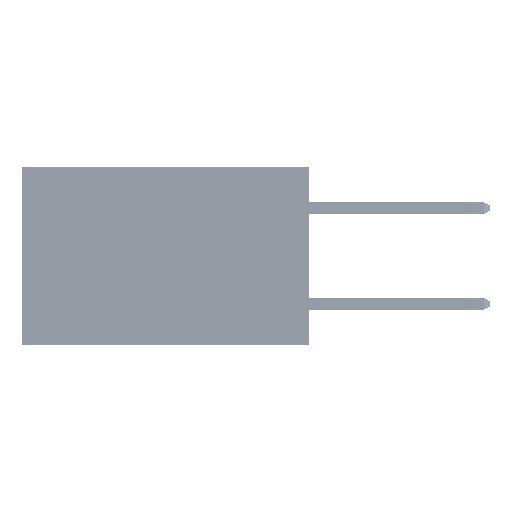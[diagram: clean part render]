
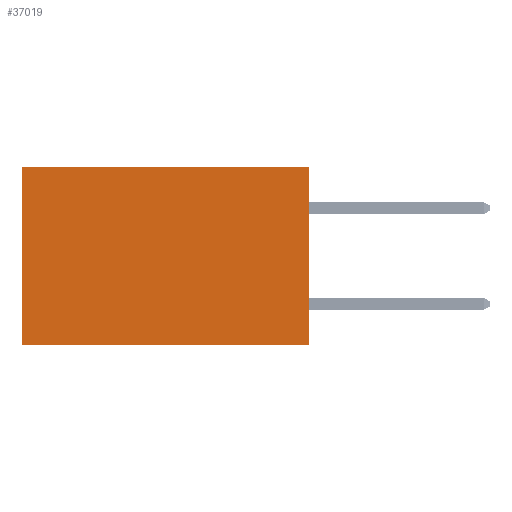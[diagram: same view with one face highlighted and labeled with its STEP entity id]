
A CAD part, left-side view. The second image highlights one B-rep face of the part: STEP entity #37019.
In plain terms, the highlighted planar face has unit normal (-1, 0, 0).
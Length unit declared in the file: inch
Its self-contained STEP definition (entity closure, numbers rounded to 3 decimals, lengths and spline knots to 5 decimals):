
#2268 = LINE ( 'NONE', #9740, #20558 ) ;
#5311 = LINE ( 'NONE', #22146, #48458 ) ;
#5512 = LINE ( 'NONE', #30117, #25499 ) ;
#9740 = CARTESIAN_POINT ( 'NONE',  ( 0.2875, 0., 0. ) ) ;
#11910 = VERTEX_POINT ( 'NONE', #40255 ) ;
#12881 = CARTESIAN_POINT ( 'NONE',  ( 0.2875, 0., 0. ) ) ;
#13113 = EDGE_CURVE ( 'NONE', #22069, #13274, #5512, .T. ) ;
#13274 = VERTEX_POINT ( 'NONE', #38878 ) ;
#13489 = EDGE_CURVE ( 'NONE', #11910, #13274, #33892, .T. ) ;
#13778 = VECTOR ( 'NONE', #17350, 39.37008 ) ;
#15370 = PLANE ( 'NONE',  #36604 ) ;
#15539 = DIRECTION ( 'NONE',  ( 1., 0., 0. ) ) ;
#16087 = EDGE_CURVE ( 'NONE', #34594, #11910, #5311, .T. ) ;
#17350 = DIRECTION ( 'NONE',  ( 0., 1., 0. ) ) ;
#20558 = VECTOR ( 'NONE', #21112, 39.37008 ) ;
#21112 = DIRECTION ( 'NONE',  ( 0., 1., 0. ) ) ;
#21831 = ORIENTED_EDGE ( 'NONE', *, *, #16087, .F. ) ;
#22069 = VERTEX_POINT ( 'NONE', #35425 ) ;
#22146 = CARTESIAN_POINT ( 'NONE',  ( 0.2875, 0., 0. ) ) ;
#24634 = FACE_OUTER_BOUND ( 'NONE', #47702, .T. ) ;
#24838 = ORIENTED_EDGE ( 'NONE', *, *, #13489, .F. ) ;
#25499 = VECTOR ( 'NONE', #42025, 39.37008 ) ;
#30117 = CARTESIAN_POINT ( 'NONE',  ( 0.2875, 0.6, 0. ) ) ;
#30265 = DIRECTION ( 'NONE',  ( 0., 0., -1. ) ) ;
#32706 = ORIENTED_EDGE ( 'NONE', *, *, #13113, .T. ) ;
#33892 = LINE ( 'NONE', #47631, #13778 ) ;
#34594 = VERTEX_POINT ( 'NONE', #12881 ) ;
#35425 = CARTESIAN_POINT ( 'NONE',  ( 0.2875, 0.6, 0. ) ) ;
#36604 = AXIS2_PLACEMENT_3D ( 'NONE', #41854, #15539, #30265 ) ;
#36730 = ORIENTED_EDGE ( 'NONE', *, *, #45154, .T. ) ;
#36893 = DIRECTION ( 'NONE',  ( 0., 0., -1. ) ) ;
#37019 = ADVANCED_FACE ( 'NONE', ( #24634 ), #15370, .F. ) ;
#38878 = CARTESIAN_POINT ( 'NONE',  ( 0.2875, 0.6, -0.37 ) ) ;
#40255 = CARTESIAN_POINT ( 'NONE',  ( 0.2875, 0., -0.37 ) ) ;
#41854 = CARTESIAN_POINT ( 'NONE',  ( 0.2875, 0., 0. ) ) ;
#42025 = DIRECTION ( 'NONE',  ( 0., 0., -1. ) ) ;
#45154 = EDGE_CURVE ( 'NONE', #34594, #22069, #2268, .T. ) ;
#47631 = CARTESIAN_POINT ( 'NONE',  ( 0.2875, 0., -0.37 ) ) ;
#47702 = EDGE_LOOP ( 'NONE', ( #32706, #24838, #21831, #36730 ) ) ;
#48458 = VECTOR ( 'NONE', #36893, 39.37008 ) ;
